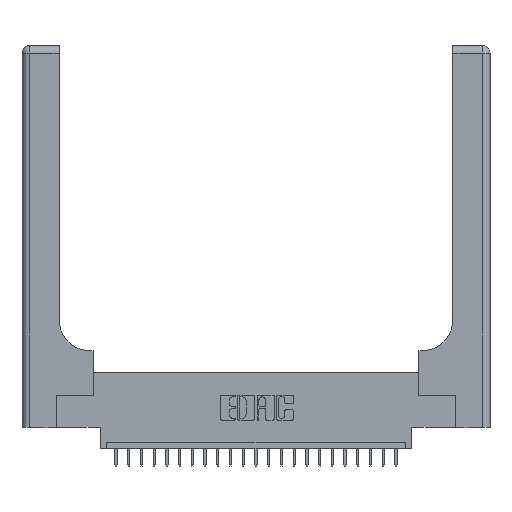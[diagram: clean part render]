
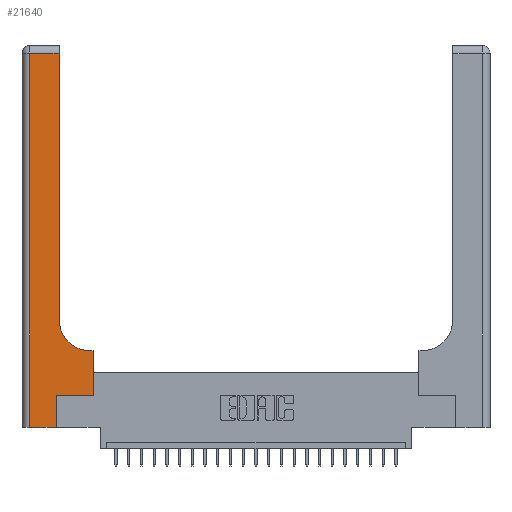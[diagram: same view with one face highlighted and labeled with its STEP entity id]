
A CAD part, top view. The second image highlights one B-rep face of the part: STEP entity #21640.
In plain terms, the highlighted planar face has unit normal (0, 0, 1).
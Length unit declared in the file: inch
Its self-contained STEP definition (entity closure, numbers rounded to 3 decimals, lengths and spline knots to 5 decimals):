
#628 = DIRECTION ( 'NONE',  ( 1., 0., 0. ) ) ;
#1128 = CARTESIAN_POINT ( 'NONE',  ( 0.5415, 0.85, 0.37 ) ) ;
#1451 = DIRECTION ( 'NONE',  ( -1., 0., 0. ) ) ;
#1539 = LINE ( 'NONE', #7314, #24299 ) ;
#1585 = EDGE_CURVE ( 'NONE', #5756, #24024, #25208, .T. ) ;
#1830 = CARTESIAN_POINT ( 'NONE',  ( 0.2915, 0.85, 0.37 ) ) ;
#1988 = EDGE_CURVE ( 'NONE', #20770, #3526, #23630, .T. ) ;
#2047 = CARTESIAN_POINT ( 'NONE',  ( 0.06, 2.94, 0.37 ) ) ;
#2077 = VECTOR ( 'NONE', #7409, 39.37008 ) ;
#2187 = CARTESIAN_POINT ( 'NONE',  ( 0.269, 0.25, 0.37 ) ) ;
#2659 = DIRECTION ( 'NONE',  ( 0., 1., 0. ) ) ;
#2780 = CARTESIAN_POINT ( 'NONE',  ( 0.269, 0., 0.37 ) ) ;
#2847 = LINE ( 'NONE', #3359, #14420 ) ;
#3013 = ORIENTED_EDGE ( 'NONE', *, *, #1988, .T. ) ;
#3158 = ORIENTED_EDGE ( 'NONE', *, *, #14945, .T. ) ;
#3359 = CARTESIAN_POINT ( 'NONE',  ( 0., 2.94, 0.37 ) ) ;
#3526 = VERTEX_POINT ( 'NONE', #16372 ) ;
#3891 = CARTESIAN_POINT ( 'NONE',  ( 0., 0., 0.37 ) ) ;
#4136 = VERTEX_POINT ( 'NONE', #14654 ) ;
#4665 = VECTOR ( 'NONE', #2659, 39.37008 ) ;
#4700 = VERTEX_POINT ( 'NONE', #2047 ) ;
#4933 = DIRECTION ( 'NONE',  ( 0., 0., -1. ) ) ;
#5717 = CARTESIAN_POINT ( 'NONE',  ( 0.5585, 0.6, 0.37 ) ) ;
#5756 = VERTEX_POINT ( 'NONE', #15590 ) ;
#5781 = EDGE_CURVE ( 'NONE', #20062, #5756, #24427, .T. ) ;
#7102 = DIRECTION ( 'NONE',  ( -1., 0., 0. ) ) ;
#7297 = EDGE_CURVE ( 'NONE', #17496, #4136, #10149, .T. ) ;
#7314 = CARTESIAN_POINT ( 'NONE',  ( 0.2915, 3., 0.37 ) ) ;
#7409 = DIRECTION ( 'NONE',  ( 0., -1., 0. ) ) ;
#8208 = ORIENTED_EDGE ( 'NONE', *, *, #7297, .T. ) ;
#8900 = FACE_OUTER_BOUND ( 'NONE', #15036, .T. ) ;
#8930 = CARTESIAN_POINT ( 'NONE',  ( 0.5585, 0.25, 0.37 ) ) ;
#10149 = LINE ( 'NONE', #2187, #19194 ) ;
#10823 = PLANE ( 'NONE',  #23454 ) ;
#10860 = DIRECTION ( 'NONE',  ( 0., 1., 0. ) ) ;
#11318 = VECTOR ( 'NONE', #21353, 39.37008 ) ;
#11498 = EDGE_CURVE ( 'NONE', #4700, #20770, #12909, .T. ) ;
#11566 = VECTOR ( 'NONE', #10860, 39.37008 ) ;
#12271 = LINE ( 'NONE', #2780, #4665 ) ;
#12629 = CARTESIAN_POINT ( 'NONE',  ( 0.2915, 0.6, 0.37 ) ) ;
#12909 = LINE ( 'NONE', #23181, #2077 ) ;
#14074 = VECTOR ( 'NONE', #18522, 39.37008 ) ;
#14420 = VECTOR ( 'NONE', #1451, 39.37008 ) ;
#14654 = CARTESIAN_POINT ( 'NONE',  ( 0.5585, 0.25, 0.37 ) ) ;
#14688 = ORIENTED_EDGE ( 'NONE', *, *, #11498, .T. ) ;
#14807 = DIRECTION ( 'NONE',  ( 0., 0., -1. ) ) ;
#14945 = EDGE_CURVE ( 'NONE', #3526, #17496, #12271, .T. ) ;
#15036 = EDGE_LOOP ( 'NONE', ( #24363, #19322, #14688, #3013, #3158, #8208, #23539, #21845, #22999 ) ) ;
#15590 = CARTESIAN_POINT ( 'NONE',  ( 0.5415, 0.6, 0.37 ) ) ;
#15789 = AXIS2_PLACEMENT_3D ( 'NONE', #1128, #14807, #628 ) ;
#15907 = DIRECTION ( 'NONE',  ( 1., 0., 0. ) ) ;
#16372 = CARTESIAN_POINT ( 'NONE',  ( 0.269, 0., 0.37 ) ) ;
#16780 = CARTESIAN_POINT ( 'NONE',  ( 0.2915, 2.94, 0.37 ) ) ;
#17152 = DIRECTION ( 'NONE',  ( 0., 1., 0. ) ) ;
#17496 = VERTEX_POINT ( 'NONE', #17589 ) ;
#17530 = CARTESIAN_POINT ( 'NONE',  ( 0.06, 0., 0.37 ) ) ;
#17589 = CARTESIAN_POINT ( 'NONE',  ( 0.269, 0.25, 0.37 ) ) ;
#18522 = DIRECTION ( 'NONE',  ( -1., 0., 0. ) ) ;
#19194 = VECTOR ( 'NONE', #15907, 39.37008 ) ;
#19322 = ORIENTED_EDGE ( 'NONE', *, *, #21674, .T. ) ;
#20062 = VERTEX_POINT ( 'NONE', #5717 ) ;
#20558 = CARTESIAN_POINT ( 'NONE',  ( 0., 3., 0.37 ) ) ;
#20729 = LINE ( 'NONE', #8930, #11566 ) ;
#20770 = VERTEX_POINT ( 'NONE', #17530 ) ;
#21353 = DIRECTION ( 'NONE',  ( 1., 0., 0. ) ) ;
#21420 = EDGE_CURVE ( 'NONE', #4136, #20062, #20729, .T. ) ;
#21640 = ADVANCED_FACE ( 'NONE', ( #8900 ), #10823, .F. ) ;
#21674 = EDGE_CURVE ( 'NONE', #22687, #4700, #2847, .T. ) ;
#21845 = ORIENTED_EDGE ( 'NONE', *, *, #5781, .T. ) ;
#22687 = VERTEX_POINT ( 'NONE', #16780 ) ;
#22892 = EDGE_CURVE ( 'NONE', #24024, #22687, #1539, .T. ) ;
#22999 = ORIENTED_EDGE ( 'NONE', *, *, #1585, .T. ) ;
#23181 = CARTESIAN_POINT ( 'NONE',  ( 0.06, 3., 0.37 ) ) ;
#23454 = AXIS2_PLACEMENT_3D ( 'NONE', #20558, #4933, #7102 ) ;
#23539 = ORIENTED_EDGE ( 'NONE', *, *, #21420, .T. ) ;
#23630 = LINE ( 'NONE', #3891, #11318 ) ;
#24024 = VERTEX_POINT ( 'NONE', #1830 ) ;
#24299 = VECTOR ( 'NONE', #17152, 39.37008 ) ;
#24363 = ORIENTED_EDGE ( 'NONE', *, *, #22892, .T. ) ;
#24427 = LINE ( 'NONE', #12629, #14074 ) ;
#25208 = CIRCLE ( 'NONE', #15789, 0.25 ) ;
